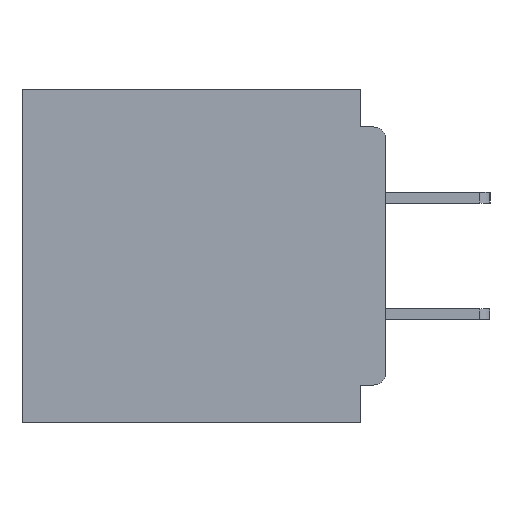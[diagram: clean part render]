
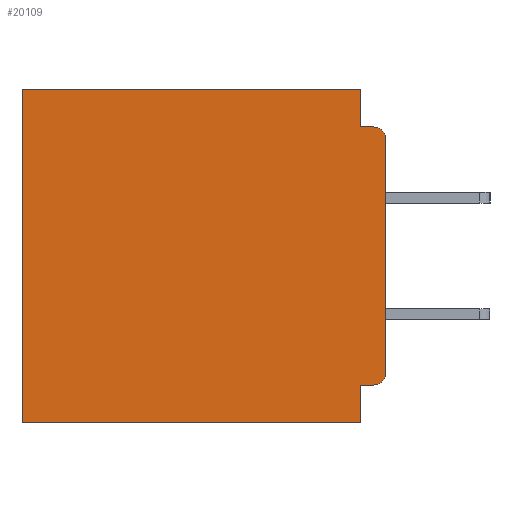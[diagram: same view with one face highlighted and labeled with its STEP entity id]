
A CAD part, left-side view. The second image highlights one B-rep face of the part: STEP entity #20109.
In plain terms, the highlighted planar face has unit normal (-1, 0, 0).
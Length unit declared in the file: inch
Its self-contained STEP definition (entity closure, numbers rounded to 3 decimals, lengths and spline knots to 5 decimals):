
#511 = VERTEX_POINT ( 'NONE', #34038 ) ;
#776 = CARTESIAN_POINT ( 'NONE',  ( 0.3, 0., -0.355 ) ) ;
#1021 = DIRECTION ( 'NONE',  ( 0., 0., -1. ) ) ;
#1725 = EDGE_CURVE ( 'NONE', #16581, #511, #29722, .T. ) ;
#2137 = CARTESIAN_POINT ( 'NONE',  ( 0.3, 0.015, -0.34 ) ) ;
#2210 = DIRECTION ( 'NONE',  ( -1., 0., 0. ) ) ;
#2394 = EDGE_CURVE ( 'NONE', #14757, #511, #20619, .T. ) ;
#2915 = CARTESIAN_POINT ( 'NONE',  ( 0.3, 0., -0.4 ) ) ;
#3552 = CARTESIAN_POINT ( 'NONE',  ( 0.3, 0.015, -0.045 ) ) ;
#4606 = ORIENTED_EDGE ( 'NONE', *, *, #41128, .F. ) ;
#4782 = VECTOR ( 'NONE', #22270, 39.37008 ) ;
#5447 = DIRECTION ( 'NONE',  ( 0., 0., -1. ) ) ;
#6480 = DIRECTION ( 'NONE',  ( 1., 0., 0. ) ) ;
#7686 = LINE ( 'NONE', #18051, #35549 ) ;
#8340 = ORIENTED_EDGE ( 'NONE', *, *, #22307, .T. ) ;
#8865 = CARTESIAN_POINT ( 'NONE',  ( 0.3, 0.437, 0. ) ) ;
#10804 = FACE_OUTER_BOUND ( 'NONE', #12118, .T. ) ;
#12088 = EDGE_CURVE ( 'NONE', #24364, #36301, #34452, .T. ) ;
#12118 = EDGE_LOOP ( 'NONE', ( #12863, #8340, #16527, #14418, #20616, #26139, #36615, #14804, #4606, #36823 ) ) ;
#12585 = VECTOR ( 'NONE', #40961, 39.37008 ) ;
#12863 = ORIENTED_EDGE ( 'NONE', *, *, #34164, .F. ) ;
#13872 = AXIS2_PLACEMENT_3D ( 'NONE', #21828, #2210, #25072 ) ;
#14418 = ORIENTED_EDGE ( 'NONE', *, *, #12088, .F. ) ;
#14445 = LINE ( 'NONE', #776, #31619 ) ;
#14757 = VERTEX_POINT ( 'NONE', #34176 ) ;
#14804 = ORIENTED_EDGE ( 'NONE', *, *, #22856, .F. ) ;
#15107 = AXIS2_PLACEMENT_3D ( 'NONE', #2137, #25004, #5447 ) ;
#15264 = DIRECTION ( 'NONE',  ( 0., 1., 0. ) ) ;
#15651 = VECTOR ( 'NONE', #15264, 39.37008 ) ;
#15808 = DIRECTION ( 'NONE',  ( 0., 0., -1. ) ) ;
#16527 = ORIENTED_EDGE ( 'NONE', *, *, #38934, .F. ) ;
#16581 = VERTEX_POINT ( 'NONE', #8865 ) ;
#16676 = CARTESIAN_POINT ( 'NONE',  ( 0.3, 0.015, -0.355 ) ) ;
#17466 = CARTESIAN_POINT ( 'NONE',  ( 0.3, 0., -0.34 ) ) ;
#18051 = CARTESIAN_POINT ( 'NONE',  ( 0.3, 0.031, -0.4 ) ) ;
#18362 = EDGE_CURVE ( 'NONE', #23858, #29619, #19697, .T. ) ;
#19697 = CIRCLE ( 'NONE', #15107, 0.015 ) ;
#19964 = DIRECTION ( 'NONE',  ( 0., 1., 0. ) ) ;
#20109 = ADVANCED_FACE ( 'NONE', ( #10804 ), #22778, .F. ) ;
#20616 = ORIENTED_EDGE ( 'NONE', *, *, #37037, .T. ) ;
#20619 = LINE ( 'NONE', #2915, #29163 ) ;
#21185 = AXIS2_PLACEMENT_3D ( 'NONE', #26009, #6480, #29230 ) ;
#21828 = CARTESIAN_POINT ( 'NONE',  ( 0.3, 0.015, -0.06 ) ) ;
#22270 = DIRECTION ( 'NONE',  ( 0., 0., -1. ) ) ;
#22296 = LINE ( 'NONE', #34561, #12585 ) ;
#22307 = EDGE_CURVE ( 'NONE', #22327, #33120, #36579, .T. ) ;
#22327 = VERTEX_POINT ( 'NONE', #34548 ) ;
#22778 = PLANE ( 'NONE',  #21185 ) ;
#22856 = EDGE_CURVE ( 'NONE', #24582, #14757, #7686, .T. ) ;
#23472 = CARTESIAN_POINT ( 'NONE',  ( 0.3, 0.031, -0.355 ) ) ;
#23858 = VERTEX_POINT ( 'NONE', #16676 ) ;
#24320 = LINE ( 'NONE', #28161, #15651 ) ;
#24364 = VERTEX_POINT ( 'NONE', #28820 ) ;
#24582 = VERTEX_POINT ( 'NONE', #23472 ) ;
#24642 = CARTESIAN_POINT ( 'NONE',  ( 0.3, 0.437, -0.4 ) ) ;
#25004 = DIRECTION ( 'NONE',  ( -1., 0., 0. ) ) ;
#25072 = DIRECTION ( 'NONE',  ( 0., 0., -1. ) ) ;
#25963 = VECTOR ( 'NONE', #15808, 39.37008 ) ;
#26009 = CARTESIAN_POINT ( 'NONE',  ( 0.3, 0., -0.4 ) ) ;
#26139 = ORIENTED_EDGE ( 'NONE', *, *, #1725, .T. ) ;
#26530 = LINE ( 'NONE', #27129, #34994 ) ;
#26898 = DIRECTION ( 'NONE',  ( 0., 1., 0. ) ) ;
#27129 = CARTESIAN_POINT ( 'NONE',  ( 0.3, 0., -0.4 ) ) ;
#28161 = CARTESIAN_POINT ( 'NONE',  ( 0.3, 0., 0. ) ) ;
#28820 = CARTESIAN_POINT ( 'NONE',  ( 0.3, 0.031, 0. ) ) ;
#29163 = VECTOR ( 'NONE', #19964, 39.37008 ) ;
#29230 = DIRECTION ( 'NONE',  ( 0., 0., -1. ) ) ;
#29619 = VERTEX_POINT ( 'NONE', #17466 ) ;
#29722 = LINE ( 'NONE', #24642, #4782 ) ;
#31619 = VECTOR ( 'NONE', #26898, 39.37008 ) ;
#33120 = VERTEX_POINT ( 'NONE', #3552 ) ;
#34038 = CARTESIAN_POINT ( 'NONE',  ( 0.3, 0.437, -0.4 ) ) ;
#34164 = EDGE_CURVE ( 'NONE', #22327, #29619, #26530, .T. ) ;
#34176 = CARTESIAN_POINT ( 'NONE',  ( 0.3, 0.031, -0.4 ) ) ;
#34452 = LINE ( 'NONE', #35099, #25963 ) ;
#34548 = CARTESIAN_POINT ( 'NONE',  ( 0.3, 0., -0.06 ) ) ;
#34561 = CARTESIAN_POINT ( 'NONE',  ( 0.3, 0., -0.045 ) ) ;
#34994 = VECTOR ( 'NONE', #1021, 39.37008 ) ;
#35099 = CARTESIAN_POINT ( 'NONE',  ( 0.3, 0.031, 0. ) ) ;
#35212 = CARTESIAN_POINT ( 'NONE',  ( 0.3, 0.031, -0.045 ) ) ;
#35549 = VECTOR ( 'NONE', #37282, 39.37008 ) ;
#36301 = VERTEX_POINT ( 'NONE', #35212 ) ;
#36579 = CIRCLE ( 'NONE', #13872, 0.015 ) ;
#36615 = ORIENTED_EDGE ( 'NONE', *, *, #2394, .F. ) ;
#36823 = ORIENTED_EDGE ( 'NONE', *, *, #18362, .T. ) ;
#37037 = EDGE_CURVE ( 'NONE', #24364, #16581, #24320, .T. ) ;
#37282 = DIRECTION ( 'NONE',  ( 0., 0., -1. ) ) ;
#38934 = EDGE_CURVE ( 'NONE', #36301, #33120, #22296, .T. ) ;
#40961 = DIRECTION ( 'NONE',  ( 0., -1., 0. ) ) ;
#41128 = EDGE_CURVE ( 'NONE', #23858, #24582, #14445, .T. ) ;
